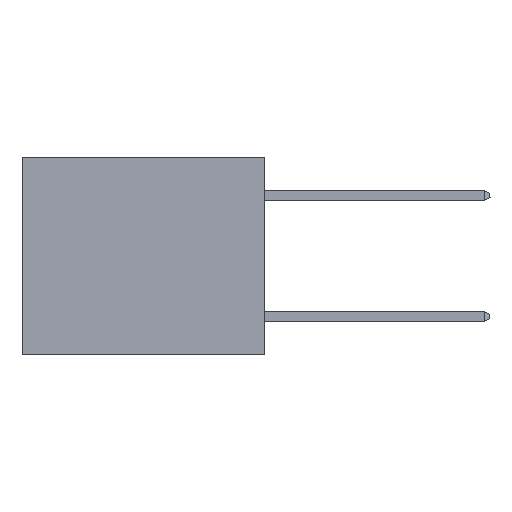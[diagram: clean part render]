
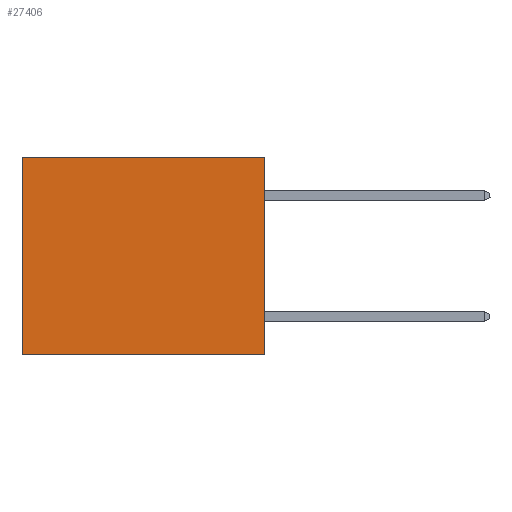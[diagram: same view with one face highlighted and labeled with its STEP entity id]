
A CAD part, left-side view. The second image highlights one B-rep face of the part: STEP entity #27406.
In plain terms, the highlighted planar face has unit normal (-1, 0, 0).
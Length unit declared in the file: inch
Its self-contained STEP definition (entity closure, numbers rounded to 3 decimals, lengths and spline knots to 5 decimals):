
#495 = CARTESIAN_POINT ( 'NONE',  ( 0.3165, 0., -0.49 ) ) ;
#608 = DIRECTION ( 'NONE',  ( 1., 0., 0. ) ) ;
#869 = EDGE_CURVE ( 'NONE', #20090, #19763, #26674, .T. ) ;
#1411 = VECTOR ( 'NONE', #17669, 39.37008 ) ;
#3257 = VERTEX_POINT ( 'NONE', #19306 ) ;
#3277 = VECTOR ( 'NONE', #21508, 39.37008 ) ;
#5257 = EDGE_CURVE ( 'NONE', #20090, #16336, #15693, .T. ) ;
#6076 = ORIENTED_EDGE ( 'NONE', *, *, #869, .T. ) ;
#11642 = CARTESIAN_POINT ( 'NONE',  ( 0.3165, 0.6, 0. ) ) ;
#12041 = CARTESIAN_POINT ( 'NONE',  ( 0.3165, 0., 0. ) ) ;
#12106 = CARTESIAN_POINT ( 'NONE',  ( 0.3165, 0.6, -0.49 ) ) ;
#12510 = FACE_OUTER_BOUND ( 'NONE', #20407, .T. ) ;
#12549 = EDGE_CURVE ( 'NONE', #16336, #3257, #17295, .T. ) ;
#12931 = EDGE_CURVE ( 'NONE', #19763, #3257, #15472, .T. ) ;
#14862 = CARTESIAN_POINT ( 'NONE',  ( 0.3165, 0., -0.49 ) ) ;
#15375 = CARTESIAN_POINT ( 'NONE',  ( 0.3165, 0., 0. ) ) ;
#15472 = LINE ( 'NONE', #12106, #3277 ) ;
#15693 = LINE ( 'NONE', #14862, #27998 ) ;
#16138 = DIRECTION ( 'NONE',  ( 0., 1., 0. ) ) ;
#16336 = VERTEX_POINT ( 'NONE', #22252 ) ;
#16724 = DIRECTION ( 'NONE',  ( 0., 0., -1. ) ) ;
#17295 = LINE ( 'NONE', #495, #19079 ) ;
#17669 = DIRECTION ( 'NONE',  ( 0., 1., 0. ) ) ;
#19014 = CARTESIAN_POINT ( 'NONE',  ( 0.3165, 0., -0.49 ) ) ;
#19079 = VECTOR ( 'NONE', #16138, 39.37008 ) ;
#19306 = CARTESIAN_POINT ( 'NONE',  ( 0.3165, 0.6, -0.49 ) ) ;
#19623 = ORIENTED_EDGE ( 'NONE', *, *, #5257, .F. ) ;
#19763 = VERTEX_POINT ( 'NONE', #11642 ) ;
#20090 = VERTEX_POINT ( 'NONE', #12041 ) ;
#20407 = EDGE_LOOP ( 'NONE', ( #22135, #21305, #19623, #6076 ) ) ;
#21305 = ORIENTED_EDGE ( 'NONE', *, *, #12549, .F. ) ;
#21508 = DIRECTION ( 'NONE',  ( 0., 0., -1. ) ) ;
#22135 = ORIENTED_EDGE ( 'NONE', *, *, #12931, .T. ) ;
#22252 = CARTESIAN_POINT ( 'NONE',  ( 0.3165, 0., -0.49 ) ) ;
#25905 = PLANE ( 'NONE',  #29113 ) ;
#26573 = DIRECTION ( 'NONE',  ( 0., 0., -1. ) ) ;
#26674 = LINE ( 'NONE', #15375, #1411 ) ;
#27406 = ADVANCED_FACE ( 'NONE', ( #12510 ), #25905, .F. ) ;
#27998 = VECTOR ( 'NONE', #26573, 39.37008 ) ;
#29113 = AXIS2_PLACEMENT_3D ( 'NONE', #19014, #608, #16724 ) ;
